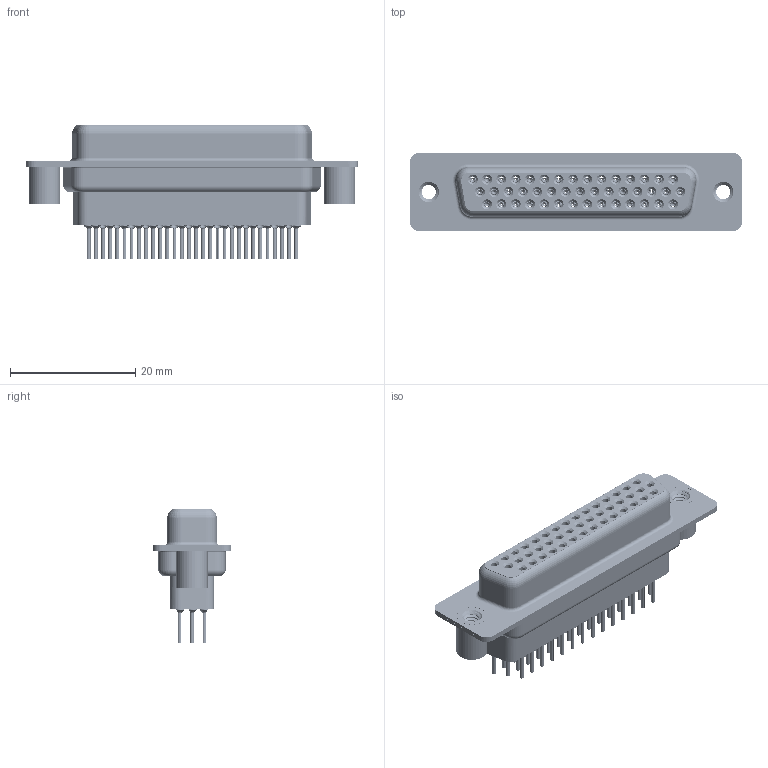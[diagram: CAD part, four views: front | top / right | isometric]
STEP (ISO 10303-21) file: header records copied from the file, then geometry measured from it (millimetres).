
FILE_DESCRIPTION (( 'STEP AP203' ), '1' );
FILE_NAME ('638-044-331-279.STEP', '2020-07-18T23:26:06', ( '' ), ( '' ), 'SwSTEP 2.0', 'SolidWorks 2020', '' );
FILE_SCHEMA (( 'CONFIG_CONTROL_DESIGN' ));
Length unit declared in the file: millimetre
Products named in the file (8): 638 Shell Front_44 Contacts; 638-044-331-279; 638 Shell Rear_44 Contacts; 638 Contact Row 2_31; 638 Contact Row 3_31; 638 Housing_44 Contacts HP; 638 Contact Row 1_31; 638 4-40 Threaded Standoff BS
Assembly tree (49 placements, depth 2):
  638-044-331-279
    638 Housing_44 Contacts HP
    638 Shell Front_44 Contacts
    638 Shell Rear_44 Contacts
    638 Contact Row 1_31  x15
    638 Contact Row 2_31  x15
    638 Contact Row 3_31  x14
    638 4-40 Threaded Standoff BS  x2
Bounding box: 53.04 x 12.6 x 21.5 mm (x, y, z)
Volume: 4079 mm3; surface area: 15540.8 mm2
Topology: 49 solids, 49 shells, 5713 faces, 14653 edges, 9137 vertices
Faces by surface type: cylinder 1609, plane 1431, torus 1113, bspline 886, cone 674
Entity records: 40302 total; most frequent: CARTESIAN_POINT 11124, DIRECTION 6021, ORIENTED_EDGE 5458, EDGE_CURVE 2729, AXIS2_PLACEMENT_3D 2532, VERTEX_POINT 1725, EDGE_LOOP 1402, CIRCLE 1384
